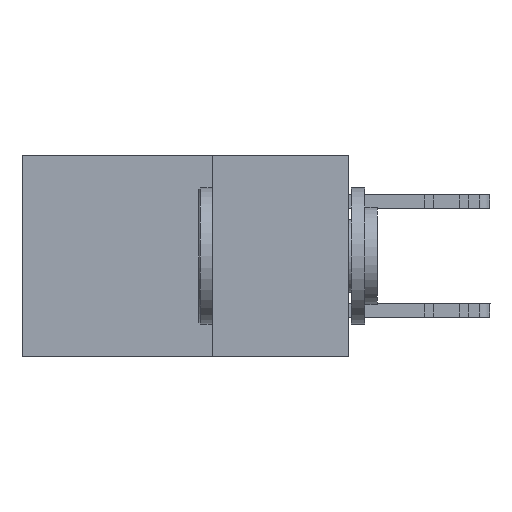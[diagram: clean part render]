
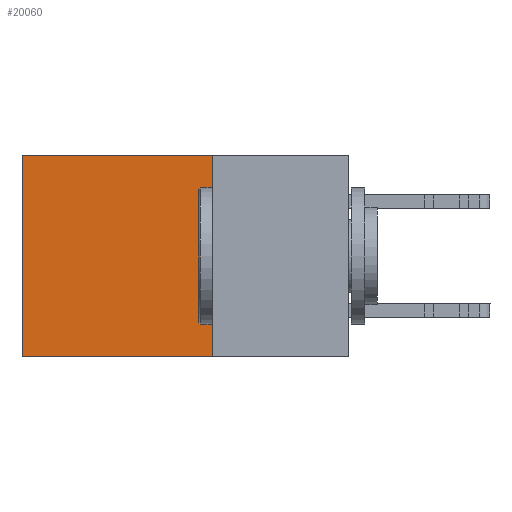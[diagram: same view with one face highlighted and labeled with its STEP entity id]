
A CAD part, left-side view. The second image highlights one B-rep face of the part: STEP entity #20060.
In plain terms, the highlighted planar face has unit normal (-1, 0, 0).
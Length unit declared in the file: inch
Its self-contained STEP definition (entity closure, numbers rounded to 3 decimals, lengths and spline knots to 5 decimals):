
#39 = DIRECTION ( 'NONE',  ( 1., 0., 0. ) ) ;
#424 = ORIENTED_EDGE ( 'NONE', *, *, #15317, .F. ) ;
#808 = CARTESIAN_POINT ( 'NONE',  ( 0.2615, 0.6, 0. ) ) ;
#936 = DIRECTION ( 'NONE',  ( 0., 0., -1. ) ) ;
#3072 = LINE ( 'NONE', #10281, #22241 ) ;
#4126 = VERTEX_POINT ( 'NONE', #20161 ) ;
#5793 = VECTOR ( 'NONE', #9167, 39.37008 ) ;
#7481 = CARTESIAN_POINT ( 'NONE',  ( 0.2615, 0.25, -0.37 ) ) ;
#8752 = ORIENTED_EDGE ( 'NONE', *, *, #8950, .T. ) ;
#8950 = EDGE_CURVE ( 'NONE', #11036, #4126, #3072, .T. ) ;
#9167 = DIRECTION ( 'NONE',  ( 0., 1., 0. ) ) ;
#9225 = DIRECTION ( 'NONE',  ( 0., 1., 0. ) ) ;
#9545 = FACE_OUTER_BOUND ( 'NONE', #16836, .T. ) ;
#9841 = LINE ( 'NONE', #20346, #19129 ) ;
#10236 = CARTESIAN_POINT ( 'NONE',  ( 0.2615, 0.25, -0.37 ) ) ;
#10281 = CARTESIAN_POINT ( 'NONE',  ( 0.2615, 0.6, -0.37 ) ) ;
#10716 = LINE ( 'NONE', #22140, #5793 ) ;
#11036 = VERTEX_POINT ( 'NONE', #808 ) ;
#11918 = CARTESIAN_POINT ( 'NONE',  ( 0.2615, 0.25, 0. ) ) ;
#12146 = DIRECTION ( 'NONE',  ( 0., 0., -1. ) ) ;
#13093 = DIRECTION ( 'NONE',  ( 0., 0., -1. ) ) ;
#14789 = ORIENTED_EDGE ( 'NONE', *, *, #20006, .T. ) ;
#15317 = EDGE_CURVE ( 'NONE', #22184, #17104, #17992, .T. ) ;
#15562 = ORIENTED_EDGE ( 'NONE', *, *, #15689, .F. ) ;
#15689 = EDGE_CURVE ( 'NONE', #17104, #4126, #9841, .T. ) ;
#16836 = EDGE_LOOP ( 'NONE', ( #8752, #15562, #424, #14789 ) ) ;
#17104 = VERTEX_POINT ( 'NONE', #20451 ) ;
#17405 = VECTOR ( 'NONE', #936, 39.37008 ) ;
#17992 = LINE ( 'NONE', #10236, #17405 ) ;
#19129 = VECTOR ( 'NONE', #9225, 39.37008 ) ;
#20006 = EDGE_CURVE ( 'NONE', #22184, #11036, #10716, .T. ) ;
#20060 = ADVANCED_FACE ( 'NONE', ( #9545 ), #20448, .F. ) ;
#20161 = CARTESIAN_POINT ( 'NONE',  ( 0.2615, 0.6, -0.37 ) ) ;
#20346 = CARTESIAN_POINT ( 'NONE',  ( 0.2615, 0.25, -0.37 ) ) ;
#20448 = PLANE ( 'NONE',  #22309 ) ;
#20451 = CARTESIAN_POINT ( 'NONE',  ( 0.2615, 0.25, -0.37 ) ) ;
#22140 = CARTESIAN_POINT ( 'NONE',  ( 0.2615, 0.25, 0. ) ) ;
#22184 = VERTEX_POINT ( 'NONE', #11918 ) ;
#22241 = VECTOR ( 'NONE', #12146, 39.37008 ) ;
#22309 = AXIS2_PLACEMENT_3D ( 'NONE', #7481, #39, #13093 ) ;
